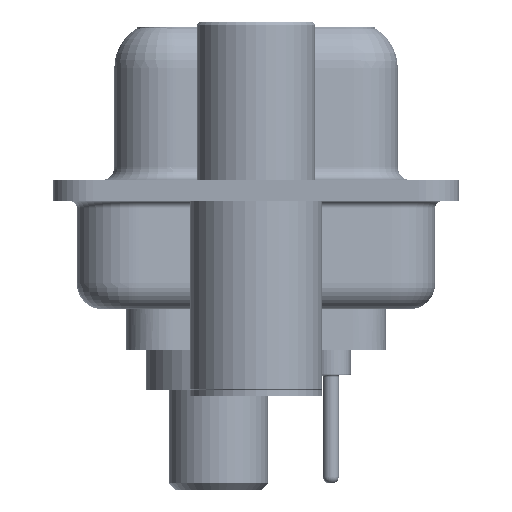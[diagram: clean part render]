
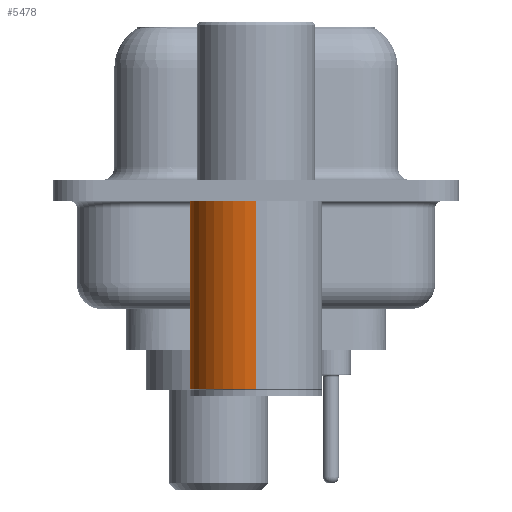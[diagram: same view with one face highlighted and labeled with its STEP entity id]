
A CAD part, left-side view. The second image highlights one B-rep face of the part: STEP entity #5478.
In plain terms, the highlighted cylindrical face has radius 2.5 mm (diameter 5 mm), a partial arc.
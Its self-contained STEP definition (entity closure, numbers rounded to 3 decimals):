
#575 = EDGE_CURVE ( 'NONE', #18171, #28104, #8510, .T. ) ;
#625 = DIRECTION ( 'NONE',  ( 0., 0., 1. ) ) ;
#1799 = AXIS2_PLACEMENT_3D ( 'NONE', #12163, #20548, #20672 ) ;
#5478 = ADVANCED_FACE ( 'NONE', ( #12896 ), #9915, .T. ) ;
#6611 = ORIENTED_EDGE ( 'NONE', *, *, #17475, .T. ) ;
#6889 = EDGE_CURVE ( 'NONE', #28104, #32039, #26159, .T. ) ;
#7754 = CARTESIAN_POINT ( 'NONE',  ( 2.5, 0., -7.525 ) ) ;
#8082 = LINE ( 'NONE', #25826, #27449 ) ;
#8141 = DIRECTION ( 'NONE',  ( 0., 0., 1. ) ) ;
#8510 = LINE ( 'NONE', #32794, #29580 ) ;
#9915 = CYLINDRICAL_SURFACE ( 'NONE', #25620, 2.5 ) ;
#12163 = CARTESIAN_POINT ( 'NONE',  ( 0., 0., -7.525 ) ) ;
#12896 = FACE_OUTER_BOUND ( 'NONE', #20440, .T. ) ;
#13347 = CARTESIAN_POINT ( 'NONE',  ( 0., 0., 0.581 ) ) ;
#13854 = EDGE_CURVE ( 'NONE', #27823, #32039, #8082, .T. ) ;
#17384 = CIRCLE ( 'NONE', #1799, 2.5 ) ;
#17475 = EDGE_CURVE ( 'NONE', #18171, #27823, #17384, .T. ) ;
#18171 = VERTEX_POINT ( 'NONE', #7754 ) ;
#18524 = DIRECTION ( 'NONE',  ( 0., 0., 1. ) ) ;
#19642 = AXIS2_PLACEMENT_3D ( 'NONE', #22692, #625, #28253 ) ;
#20440 = EDGE_LOOP ( 'NONE', ( #6611, #23652, #26044, #32759 ) ) ;
#20548 = DIRECTION ( 'NONE',  ( 0., 0., 1. ) ) ;
#20672 = DIRECTION ( 'NONE',  ( 1., 0., 0. ) ) ;
#20836 = CARTESIAN_POINT ( 'NONE',  ( 2.5, 0., -0.4 ) ) ;
#22692 = CARTESIAN_POINT ( 'NONE',  ( 0., 0., -0.4 ) ) ;
#23030 = DIRECTION ( 'NONE',  ( 0., 0., 1. ) ) ;
#23652 = ORIENTED_EDGE ( 'NONE', *, *, #13854, .T. ) ;
#24050 = DIRECTION ( 'NONE',  ( 1., 0., 0. ) ) ;
#25086 = CARTESIAN_POINT ( 'NONE',  ( -2.5, 0., -7.525 ) ) ;
#25620 = AXIS2_PLACEMENT_3D ( 'NONE', #13347, #18524, #24050 ) ;
#25826 = CARTESIAN_POINT ( 'NONE',  ( -2.5, 0., 0.581 ) ) ;
#26044 = ORIENTED_EDGE ( 'NONE', *, *, #6889, .F. ) ;
#26159 = CIRCLE ( 'NONE', #19642, 2.5 ) ;
#27449 = VECTOR ( 'NONE', #23030, 1000. ) ;
#27823 = VERTEX_POINT ( 'NONE', #25086 ) ;
#28104 = VERTEX_POINT ( 'NONE', #20836 ) ;
#28253 = DIRECTION ( 'NONE',  ( 1., 0., 0. ) ) ;
#29580 = VECTOR ( 'NONE', #8141, 1000. ) ;
#29975 = CARTESIAN_POINT ( 'NONE',  ( -2.5, 0., -0.4 ) ) ;
#32039 = VERTEX_POINT ( 'NONE', #29975 ) ;
#32759 = ORIENTED_EDGE ( 'NONE', *, *, #575, .F. ) ;
#32794 = CARTESIAN_POINT ( 'NONE',  ( 2.5, 0., 0.581 ) ) ;
